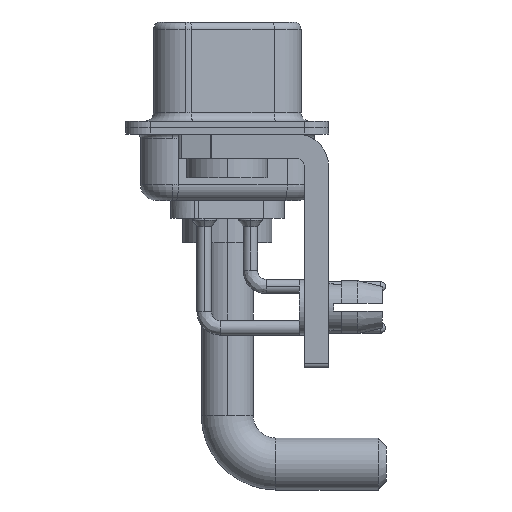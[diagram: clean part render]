
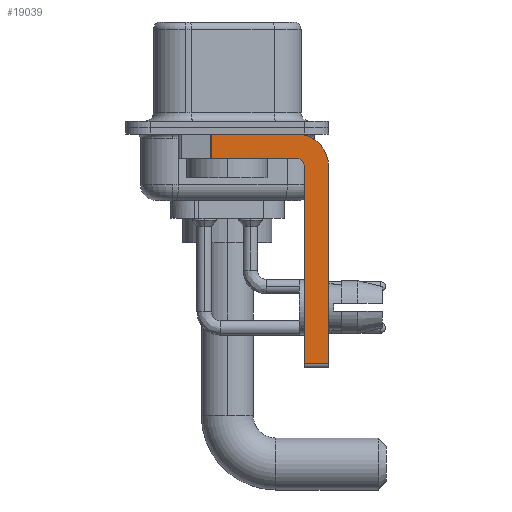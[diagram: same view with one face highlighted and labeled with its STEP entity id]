
A CAD part, left-side view. The second image highlights one B-rep face of the part: STEP entity #19039.
In plain terms, the highlighted planar face has unit normal (-1, 0, 0).
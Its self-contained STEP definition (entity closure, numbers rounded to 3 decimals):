
#18 = CARTESIAN_POINT ( 'NONE',  ( -2.9, -4.25, -2.4 ) ) ;
#174 = EDGE_CURVE ( 'NONE', #18496, #25022, #2929, .T. ) ;
#206 = EDGE_CURVE ( 'NONE', #15373, #18496, #19065, .T. ) ;
#233 = VECTOR ( 'NONE', #8807, 1000. ) ;
#867 = DIRECTION ( 'NONE',  ( 1., 0., 0. ) ) ;
#1211 = CIRCLE ( 'NONE', #9951, 0.5 ) ;
#1468 = VERTEX_POINT ( 'NONE', #6957 ) ;
#1870 = CARTESIAN_POINT ( 'NONE',  ( -2.9, 3., -0.4 ) ) ;
#2792 = CARTESIAN_POINT ( 'NONE',  ( -2.9, -4.25, -2.4 ) ) ;
#2929 = LINE ( 'NONE', #16593, #9425 ) ;
#3012 = FACE_OUTER_BOUND ( 'NONE', #27418, .T. ) ;
#3213 = DIRECTION ( 'NONE',  ( 0., 0., -1. ) ) ;
#3380 = VERTEX_POINT ( 'NONE', #19267 ) ;
#4000 = CARTESIAN_POINT ( 'NONE',  ( -2.9, -4.75, -14.8 ) ) ;
#4618 = VECTOR ( 'NONE', #10189, 1000. ) ;
#4817 = EDGE_CURVE ( 'NONE', #3380, #15373, #21716, .T. ) ;
#5454 = LINE ( 'NONE', #14231, #11177 ) ;
#5778 = ORIENTED_EDGE ( 'NONE', *, *, #16308, .T. ) ;
#6200 = VECTOR ( 'NONE', #8368, 1000. ) ;
#6957 = CARTESIAN_POINT ( 'NONE',  ( -2.9, -4.75, -2.4 ) ) ;
#7378 = VERTEX_POINT ( 'NONE', #27160 ) ;
#8086 = LINE ( 'NONE', #27945, #6200 ) ;
#8368 = DIRECTION ( 'NONE',  ( 0., 0., -1. ) ) ;
#8807 = DIRECTION ( 'NONE',  ( 0., -1., 0. ) ) ;
#8813 = DIRECTION ( 'NONE',  ( -1., 0., 0. ) ) ;
#9350 = VERTEX_POINT ( 'NONE', #16913 ) ;
#9425 = VECTOR ( 'NONE', #27392, 1000. ) ;
#9682 = ORIENTED_EDGE ( 'NONE', *, *, #206, .F. ) ;
#9702 = EDGE_CURVE ( 'NONE', #1468, #9350, #1211, .T. ) ;
#9951 = AXIS2_PLACEMENT_3D ( 'NONE', #18, #8813, #17709 ) ;
#10020 = AXIS2_PLACEMENT_3D ( 'NONE', #18271, #867, #20572 ) ;
#10189 = DIRECTION ( 'NONE',  ( 0., 0., 1. ) ) ;
#10305 = ORIENTED_EDGE ( 'NONE', *, *, #12965, .F. ) ;
#10773 = VECTOR ( 'NONE', #13103, 1000. ) ;
#11177 = VECTOR ( 'NONE', #11797, 1000. ) ;
#11241 = LINE ( 'NONE', #20002, #233 ) ;
#11797 = DIRECTION ( 'NONE',  ( 0., 1., 0. ) ) ;
#12965 = EDGE_CURVE ( 'NONE', #9350, #16986, #5454, .T. ) ;
#13103 = DIRECTION ( 'NONE',  ( 0., -1., 0. ) ) ;
#14231 = CARTESIAN_POINT ( 'NONE',  ( -2.9, -4.25, -1.9 ) ) ;
#14431 = ORIENTED_EDGE ( 'NONE', *, *, #24904, .F. ) ;
#14746 = CARTESIAN_POINT ( 'NONE',  ( -2.9, 0.978, -1.9 ) ) ;
#15373 = VERTEX_POINT ( 'NONE', #23687 ) ;
#16055 = EDGE_CURVE ( 'NONE', #3380, #16986, #8086, .T. ) ;
#16308 = EDGE_CURVE ( 'NONE', #7378, #25022, #11241, .T. ) ;
#16593 = CARTESIAN_POINT ( 'NONE',  ( -2.9, -6.25, -2.4 ) ) ;
#16913 = CARTESIAN_POINT ( 'NONE',  ( -2.9, -4.25, -1.9 ) ) ;
#16986 = VERTEX_POINT ( 'NONE', #14746 ) ;
#17709 = DIRECTION ( 'NONE',  ( 0., 0., 1. ) ) ;
#18271 = CARTESIAN_POINT ( 'NONE',  ( -2.9, -4.25, -2.4 ) ) ;
#18496 = VERTEX_POINT ( 'NONE', #26539 ) ;
#18831 = PLANE ( 'NONE',  #10020 ) ;
#18951 = CARTESIAN_POINT ( 'NONE',  ( -2.9, -6.25, -14.55 ) ) ;
#19039 = ADVANCED_FACE ( 'NONE', ( #3012 ), #18831, .F. ) ;
#19065 = CIRCLE ( 'NONE', #26449, 2. ) ;
#19241 = LINE ( 'NONE', #4000, #4618 ) ;
#19267 = CARTESIAN_POINT ( 'NONE',  ( -2.9, 0.978, -0.4 ) ) ;
#19956 = ORIENTED_EDGE ( 'NONE', *, *, #9702, .F. ) ;
#20002 = CARTESIAN_POINT ( 'NONE',  ( -2.9, -4.25, -14.55 ) ) ;
#20333 = DIRECTION ( 'NONE',  ( 1., 0., 0. ) ) ;
#20572 = DIRECTION ( 'NONE',  ( 0., 0., -1. ) ) ;
#21716 = LINE ( 'NONE', #1870, #10773 ) ;
#22360 = ORIENTED_EDGE ( 'NONE', *, *, #16055, .T. ) ;
#22427 = ORIENTED_EDGE ( 'NONE', *, *, #4817, .F. ) ;
#23687 = CARTESIAN_POINT ( 'NONE',  ( -2.9, -4.25, -0.4 ) ) ;
#24904 = EDGE_CURVE ( 'NONE', #7378, #1468, #19241, .T. ) ;
#25022 = VERTEX_POINT ( 'NONE', #18951 ) ;
#25691 = ORIENTED_EDGE ( 'NONE', *, *, #174, .F. ) ;
#26449 = AXIS2_PLACEMENT_3D ( 'NONE', #2792, #20333, #3213 ) ;
#26539 = CARTESIAN_POINT ( 'NONE',  ( -2.9, -6.25, -2.4 ) ) ;
#27160 = CARTESIAN_POINT ( 'NONE',  ( -2.9, -4.75, -14.55 ) ) ;
#27392 = DIRECTION ( 'NONE',  ( 0., 0., -1. ) ) ;
#27418 = EDGE_LOOP ( 'NONE', ( #22427, #22360, #10305, #19956, #14431, #5778, #25691, #9682 ) ) ;
#27945 = CARTESIAN_POINT ( 'NONE',  ( -2.9, 0.978, -1.9 ) ) ;
